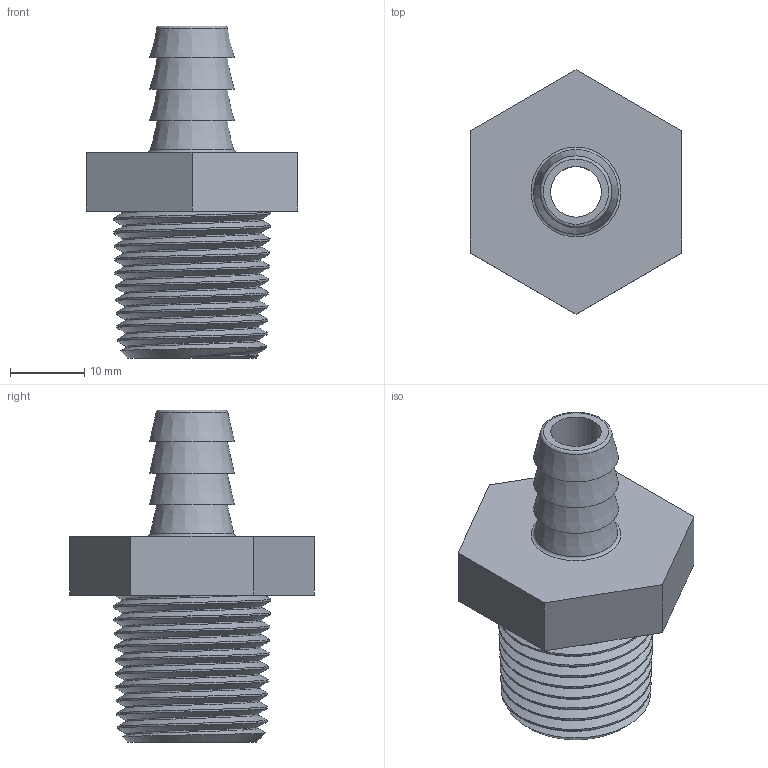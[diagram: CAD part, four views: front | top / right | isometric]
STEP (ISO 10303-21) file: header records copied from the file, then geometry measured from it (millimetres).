
FILE_DESCRIPTION(/* description */ ('STEP AP203'),/* implementation_level */ '2;1');
FILE_NAME(/* name */ 'Hose Fitting Printable.stp',/* time_stamp */ '2021-02-15T11:27:13-06:00',/* author */ ('johne'),/* organization */ (''),/* preprocessor_version */ 'ST-DEVELOPER v18',/* originating_system */ 'Autodesk Inventor 2020',/* authorisation */ '');
FILE_SCHEMA (('AUTOMOTIVE_DESIGN { 1 0 10303 214 3 1 1 }'));
Length unit declared in the file: inch
Products named in the file (1): Barbed Hose Fitting
Bounding box: 28.57 x 33 x 44.85 mm (x, y, z)
Volume: 8927 mm3; surface area: 6135.8 mm2
Topology: 1 solids, 1 shells, 39 faces, 108 edges, 76 vertices
Faces by surface type: cone 19, plane 13, bspline 3, torus 2, cylinder 2
Full cylindrical faces by diameter (mm): 6.858 x1, 13.868 x1
Entity records: 7345 total; most frequent: CARTESIAN_POINT 6319, ORIENTED_EDGE 216, DIRECTION 188, EDGE_CURVE 108, VERTEX_POINT 76, AXIS2_PLACEMENT_3D 75, EDGE_LOOP 46, FACE_OUTER_BOUND 39
